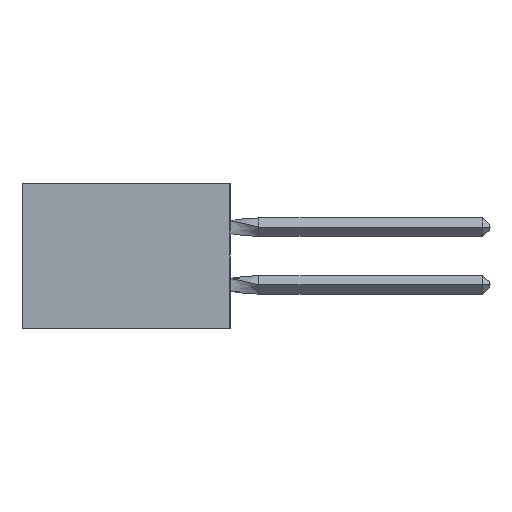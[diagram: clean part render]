
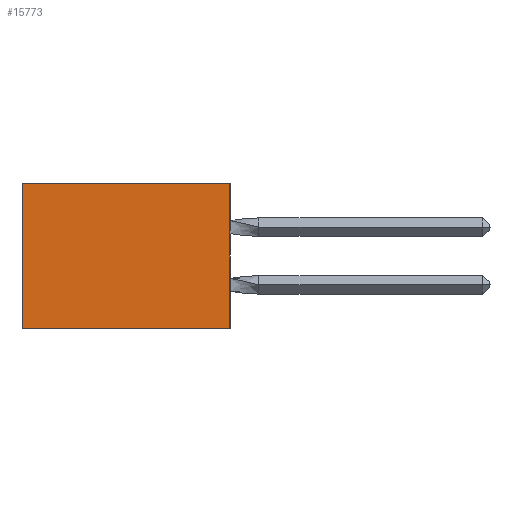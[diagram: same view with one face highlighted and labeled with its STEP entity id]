
A CAD part, left-side view. The second image highlights one B-rep face of the part: STEP entity #15773.
In plain terms, the highlighted planar face has unit normal (-1, 0, 0).
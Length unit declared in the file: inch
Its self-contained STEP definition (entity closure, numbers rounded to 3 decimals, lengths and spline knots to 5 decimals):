
#1597 = DIRECTION ( 'NONE',  ( 0., 0., -1. ) ) ;
#2933 = VERTEX_POINT ( 'NONE', #39755 ) ;
#4851 = VERTEX_POINT ( 'NONE', #30467 ) ;
#5883 = FACE_OUTER_BOUND ( 'NONE', #12889, .T. ) ;
#8100 = EDGE_CURVE ( 'NONE', #41368, #2933, #31240, .T. ) ;
#8211 = CARTESIAN_POINT ( 'NONE',  ( 0.305, 0., -0.5 ) ) ;
#8326 = ORIENTED_EDGE ( 'NONE', *, *, #18964, .T. ) ;
#9034 = LINE ( 'NONE', #30097, #27821 ) ;
#10600 = DIRECTION ( 'NONE',  ( 0., 1., 0. ) ) ;
#11628 = DIRECTION ( 'NONE',  ( 0., 0., -1. ) ) ;
#12481 = VERTEX_POINT ( 'NONE', #30533 ) ;
#12854 = CARTESIAN_POINT ( 'NONE',  ( 0.305, 0., 0. ) ) ;
#12889 = EDGE_LOOP ( 'NONE', ( #8326, #38611, #31334, #32703 ) ) ;
#14154 = CARTESIAN_POINT ( 'NONE',  ( 0.305, 0., 0. ) ) ;
#14695 = CARTESIAN_POINT ( 'NONE',  ( 0.305, 0., -0.5 ) ) ;
#15773 = ADVANCED_FACE ( 'NONE', ( #5883 ), #17809, .F. ) ;
#15791 = LINE ( 'NONE', #40137, #24883 ) ;
#17809 = PLANE ( 'NONE',  #41641 ) ;
#18964 = EDGE_CURVE ( 'NONE', #12481, #4851, #9034, .T. ) ;
#24441 = EDGE_CURVE ( 'NONE', #2933, #4851, #15791, .T. ) ;
#24883 = VECTOR ( 'NONE', #31326, 39.37008 ) ;
#27821 = VECTOR ( 'NONE', #39709, 39.37008 ) ;
#30097 = CARTESIAN_POINT ( 'NONE',  ( 0.305, 0.72, -0.5 ) ) ;
#30467 = CARTESIAN_POINT ( 'NONE',  ( 0.305, 0.72, -0.5 ) ) ;
#30533 = CARTESIAN_POINT ( 'NONE',  ( 0.305, 0.72, 0. ) ) ;
#31240 = LINE ( 'NONE', #14695, #33838 ) ;
#31326 = DIRECTION ( 'NONE',  ( 0., 1., 0. ) ) ;
#31334 = ORIENTED_EDGE ( 'NONE', *, *, #8100, .F. ) ;
#32698 = VECTOR ( 'NONE', #10600, 39.37008 ) ;
#32703 = ORIENTED_EDGE ( 'NONE', *, *, #33051, .T. ) ;
#33051 = EDGE_CURVE ( 'NONE', #41368, #12481, #37783, .T. ) ;
#33763 = DIRECTION ( 'NONE',  ( 1., 0., 0. ) ) ;
#33838 = VECTOR ( 'NONE', #1597, 39.37008 ) ;
#37783 = LINE ( 'NONE', #14154, #32698 ) ;
#38611 = ORIENTED_EDGE ( 'NONE', *, *, #24441, .F. ) ;
#39709 = DIRECTION ( 'NONE',  ( 0., 0., -1. ) ) ;
#39755 = CARTESIAN_POINT ( 'NONE',  ( 0.305, 0., -0.5 ) ) ;
#40137 = CARTESIAN_POINT ( 'NONE',  ( 0.305, 0., -0.5 ) ) ;
#41368 = VERTEX_POINT ( 'NONE', #12854 ) ;
#41641 = AXIS2_PLACEMENT_3D ( 'NONE', #8211, #33763, #11628 ) ;
